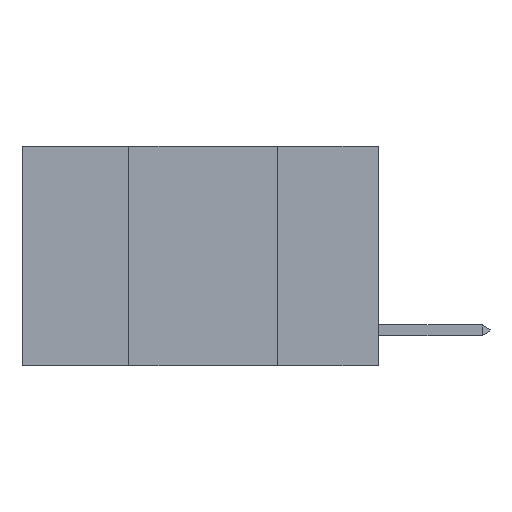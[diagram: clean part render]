
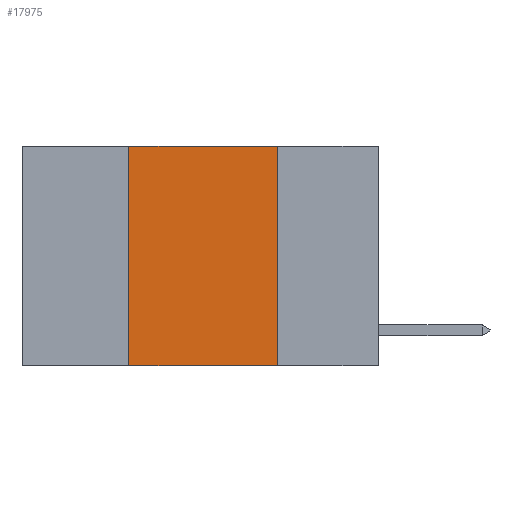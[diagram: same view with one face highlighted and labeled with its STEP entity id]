
A CAD part, left-side view. The second image highlights one B-rep face of the part: STEP entity #17975.
In plain terms, the highlighted planar face has unit normal (-1, 0, 0).
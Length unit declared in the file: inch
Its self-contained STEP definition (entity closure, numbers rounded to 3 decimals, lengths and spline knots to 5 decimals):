
#1366 = CARTESIAN_POINT ( 'NONE',  ( 0., 0.6, -0.37 ) ) ;
#1651 = DIRECTION ( 'NONE',  ( 1., 0., 0. ) ) ;
#2601 = CARTESIAN_POINT ( 'NONE',  ( 0., 0.6, 0. ) ) ;
#2875 = DIRECTION ( 'NONE',  ( 0., -1., 0. ) ) ;
#3736 = VECTOR ( 'NONE', #8643, 39.37008 ) ;
#3827 = FACE_OUTER_BOUND ( 'NONE', #12670, .T. ) ;
#4095 = CARTESIAN_POINT ( 'NONE',  ( 0., 0.17, -0.37 ) ) ;
#4152 = ORIENTED_EDGE ( 'NONE', *, *, #16524, .T. ) ;
#4526 = LINE ( 'NONE', #9453, #11216 ) ;
#4837 = VERTEX_POINT ( 'NONE', #18400 ) ;
#5338 = ORIENTED_EDGE ( 'NONE', *, *, #17171, .F. ) ;
#5974 = VECTOR ( 'NONE', #2875, 39.37008 ) ;
#6157 = PLANE ( 'NONE',  #14856 ) ;
#6471 = VECTOR ( 'NONE', #8845, 39.37008 ) ;
#6932 = LINE ( 'NONE', #16443, #6471 ) ;
#7217 = ORIENTED_EDGE ( 'NONE', *, *, #10029, .F. ) ;
#7273 = LINE ( 'NONE', #2601, #3736 ) ;
#8017 = EDGE_CURVE ( 'NONE', #14788, #9393, #4526, .T. ) ;
#8280 = VERTEX_POINT ( 'NONE', #4095 ) ;
#8643 = DIRECTION ( 'NONE',  ( 0., -1., 0. ) ) ;
#8845 = DIRECTION ( 'NONE',  ( 0., 0., -1. ) ) ;
#9393 = VERTEX_POINT ( 'NONE', #10004 ) ;
#9453 = CARTESIAN_POINT ( 'NONE',  ( 0., 0.42, 0. ) ) ;
#10004 = CARTESIAN_POINT ( 'NONE',  ( 0., 0.42, 0. ) ) ;
#10029 = EDGE_CURVE ( 'NONE', #9393, #4837, #7273, .T. ) ;
#10781 = CARTESIAN_POINT ( 'NONE',  ( 0., 0.6, 0. ) ) ;
#11216 = VECTOR ( 'NONE', #15679, 39.37008 ) ;
#12342 = DIRECTION ( 'NONE',  ( 0., 0., -1. ) ) ;
#12670 = EDGE_LOOP ( 'NONE', ( #5338, #7217, #15393, #4152 ) ) ;
#14788 = VERTEX_POINT ( 'NONE', #15304 ) ;
#14856 = AXIS2_PLACEMENT_3D ( 'NONE', #10781, #1651, #12342 ) ;
#15304 = CARTESIAN_POINT ( 'NONE',  ( 0., 0.42, -0.37 ) ) ;
#15393 = ORIENTED_EDGE ( 'NONE', *, *, #8017, .F. ) ;
#15679 = DIRECTION ( 'NONE',  ( 0., 0., 1. ) ) ;
#16443 = CARTESIAN_POINT ( 'NONE',  ( 0., 0.17, 0. ) ) ;
#16524 = EDGE_CURVE ( 'NONE', #14788, #8280, #18187, .T. ) ;
#17171 = EDGE_CURVE ( 'NONE', #4837, #8280, #6932, .T. ) ;
#17975 = ADVANCED_FACE ( 'NONE', ( #3827 ), #6157, .F. ) ;
#18187 = LINE ( 'NONE', #1366, #5974 ) ;
#18400 = CARTESIAN_POINT ( 'NONE',  ( 0., 0.17, 0. ) ) ;
